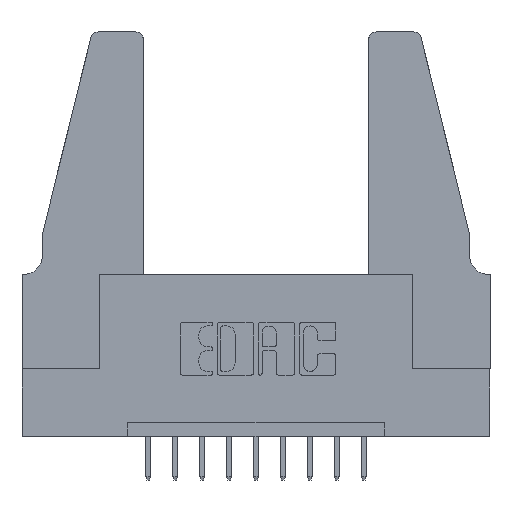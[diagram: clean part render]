
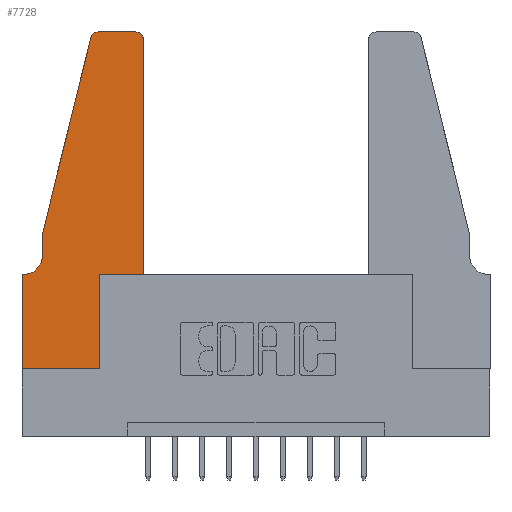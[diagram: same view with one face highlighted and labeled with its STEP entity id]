
A CAD part, top view. The second image highlights one B-rep face of the part: STEP entity #7728.
In plain terms, the highlighted planar face has unit normal (0, 0, 1).
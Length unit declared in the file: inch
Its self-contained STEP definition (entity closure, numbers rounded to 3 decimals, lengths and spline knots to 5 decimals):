
#264 = LINE ( 'NONE', #12592, #4677 ) ;
#553 = AXIS2_PLACEMENT_3D ( 'NONE', #3052, #13260, #12373 ) ;
#687 = CARTESIAN_POINT ( 'NONE',  ( 0.0755, 0.35, 0.37 ) ) ;
#752 = DIRECTION ( 'NONE',  ( 1., 0., 0. ) ) ;
#767 = EDGE_CURVE ( 'NONE', #12014, #10453, #8847, .T. ) ;
#800 = DIRECTION ( 'NONE',  ( -1., 0., 0. ) ) ;
#959 = CIRCLE ( 'NONE', #2116, 0.03 ) ;
#1011 = CIRCLE ( 'NONE', #4872, 0.07 ) ;
#1064 = EDGE_CURVE ( 'NONE', #10390, #3159, #1011, .T. ) ;
#1128 = DIRECTION ( 'NONE',  ( 0., -1., 0. ) ) ;
#1239 = LINE ( 'NONE', #7819, #7408 ) ;
#1269 = EDGE_CURVE ( 'NONE', #4932, #11868, #3289, .T. ) ;
#1440 = VERTEX_POINT ( 'NONE', #8044 ) ;
#1681 = CARTESIAN_POINT ( 'NONE',  ( 0.0755, 0.5, 0.37 ) ) ;
#1731 = CARTESIAN_POINT ( 'NONE',  ( 0.284, 1.25, 0.37 ) ) ;
#1880 = ORIENTED_EDGE ( 'NONE', *, *, #13089, .T. ) ;
#1956 = EDGE_LOOP ( 'NONE', ( #6369, #12515, #7889, #10218, #8423, #2239, #7004, #12622, #2029, #1880, #2650, #7064 ) ) ;
#2029 = ORIENTED_EDGE ( 'NONE', *, *, #767, .T. ) ;
#2116 = AXIS2_PLACEMENT_3D ( 'NONE', #11797, #7597, #5550 ) ;
#2181 = DIRECTION ( 'NONE',  ( -1., 0., 0. ) ) ;
#2197 = EDGE_CURVE ( 'NONE', #4420, #4932, #9110, .T. ) ;
#2239 = ORIENTED_EDGE ( 'NONE', *, *, #7459, .T. ) ;
#2402 = LINE ( 'NONE', #2996, #12464 ) ;
#2503 = VERTEX_POINT ( 'NONE', #6435 ) ;
#2626 = FACE_OUTER_BOUND ( 'NONE', #1956, .T. ) ;
#2650 = ORIENTED_EDGE ( 'NONE', *, *, #4150, .T. ) ;
#2946 = EDGE_CURVE ( 'NONE', #3997, #10234, #959, .T. ) ;
#2996 = CARTESIAN_POINT ( 'NONE',  ( 0.2605, 1.25, 0.37 ) ) ;
#3052 = CARTESIAN_POINT ( 'NONE',  ( 0.284, 1.22, 0.37 ) ) ;
#3159 = VERTEX_POINT ( 'NONE', #6790 ) ;
#3221 = CARTESIAN_POINT ( 'NONE',  ( 0.0055, 0.42, 0.37 ) ) ;
#3289 = LINE ( 'NONE', #1681, #3919 ) ;
#3467 = DIRECTION ( 'NONE',  ( 0., 1., 0. ) ) ;
#3749 = DIRECTION ( 'NONE',  ( 1., 0., 0. ) ) ;
#3885 = LINE ( 'NONE', #3972, #10053 ) ;
#3919 = VECTOR ( 'NONE', #4804, 39.37008 ) ;
#3972 = CARTESIAN_POINT ( 'NONE',  ( 0., 0., 0.37 ) ) ;
#3997 = VERTEX_POINT ( 'NONE', #8979 ) ;
#4150 = EDGE_CURVE ( 'NONE', #1440, #3997, #264, .T. ) ;
#4194 = PLANE ( 'NONE',  #8850 ) ;
#4245 = DIRECTION ( 'NONE',  ( 0., 0., -1. ) ) ;
#4420 = VERTEX_POINT ( 'NONE', #1731 ) ;
#4478 = EDGE_CURVE ( 'NONE', #11868, #10390, #1239, .T. ) ;
#4579 = EDGE_CURVE ( 'NONE', #10234, #4420, #2402, .T. ) ;
#4677 = VECTOR ( 'NONE', #8493, 39.37008 ) ;
#4792 = VECTOR ( 'NONE', #1128, 39.37008 ) ;
#4804 = DIRECTION ( 'NONE',  ( -0.239, -0.971, 0. ) ) ;
#4859 = CARTESIAN_POINT ( 'NONE',  ( 0.2865, 0., 0.37 ) ) ;
#4872 = AXIS2_PLACEMENT_3D ( 'NONE', #3221, #4245, #2181 ) ;
#4932 = VERTEX_POINT ( 'NONE', #9195 ) ;
#5506 = CARTESIAN_POINT ( 'NONE',  ( 0.0755, 0.42, 0.37 ) ) ;
#5550 = DIRECTION ( 'NONE',  ( 1., 0., 0. ) ) ;
#6369 = ORIENTED_EDGE ( 'NONE', *, *, #4579, .T. ) ;
#6435 = CARTESIAN_POINT ( 'NONE',  ( 0., 0., 0.37 ) ) ;
#6579 = EDGE_CURVE ( 'NONE', #7471, #2503, #8677, .T. ) ;
#6692 = CARTESIAN_POINT ( 'NONE',  ( 0.2865, 0.35, 0.37 ) ) ;
#6694 = LINE ( 'NONE', #11134, #9611 ) ;
#6790 = CARTESIAN_POINT ( 'NONE',  ( 0.0055, 0.35, 0.37 ) ) ;
#7004 = ORIENTED_EDGE ( 'NONE', *, *, #6579, .T. ) ;
#7064 = ORIENTED_EDGE ( 'NONE', *, *, #2946, .T. ) ;
#7071 = CARTESIAN_POINT ( 'NONE',  ( 0.4205, 1.25, 0.37 ) ) ;
#7408 = VECTOR ( 'NONE', #9173, 39.37008 ) ;
#7459 = EDGE_CURVE ( 'NONE', #3159, #7471, #12400, .T. ) ;
#7471 = VERTEX_POINT ( 'NONE', #11082 ) ;
#7597 = DIRECTION ( 'NONE',  ( 0., 0., 1. ) ) ;
#7685 = EDGE_CURVE ( 'NONE', #2503, #12014, #3885, .T. ) ;
#7728 = ADVANCED_FACE ( 'NONE', ( #2626 ), #4194, .T. ) ;
#7819 = CARTESIAN_POINT ( 'NONE',  ( 0.0755, 0.5, 0.37 ) ) ;
#7889 = ORIENTED_EDGE ( 'NONE', *, *, #1269, .T. ) ;
#8044 = CARTESIAN_POINT ( 'NONE',  ( 0.4505, 0.35, 0.37 ) ) ;
#8134 = VECTOR ( 'NONE', #11125, 39.37008 ) ;
#8423 = ORIENTED_EDGE ( 'NONE', *, *, #1064, .T. ) ;
#8493 = DIRECTION ( 'NONE',  ( 0., 1., 0. ) ) ;
#8677 = LINE ( 'NONE', #10558, #4792 ) ;
#8847 = LINE ( 'NONE', #6692, #10595 ) ;
#8850 = AXIS2_PLACEMENT_3D ( 'NONE', #10308, #13415, #11478 ) ;
#8979 = CARTESIAN_POINT ( 'NONE',  ( 0.4505, 1.22, 0.37 ) ) ;
#9110 = CIRCLE ( 'NONE', #553, 0.03 ) ;
#9173 = DIRECTION ( 'NONE',  ( 0., -1., 0. ) ) ;
#9195 = CARTESIAN_POINT ( 'NONE',  ( 0.25487, 1.22718, 0.37 ) ) ;
#9611 = VECTOR ( 'NONE', #3749, 39.37008 ) ;
#10053 = VECTOR ( 'NONE', #752, 39.37008 ) ;
#10218 = ORIENTED_EDGE ( 'NONE', *, *, #4478, .T. ) ;
#10234 = VERTEX_POINT ( 'NONE', #7071 ) ;
#10308 = CARTESIAN_POINT ( 'NONE',  ( 0., 0.35, 0.37 ) ) ;
#10390 = VERTEX_POINT ( 'NONE', #5506 ) ;
#10453 = VERTEX_POINT ( 'NONE', #10675 ) ;
#10558 = CARTESIAN_POINT ( 'NONE',  ( 0., 0., 0.37 ) ) ;
#10595 = VECTOR ( 'NONE', #3467, 39.37008 ) ;
#10675 = CARTESIAN_POINT ( 'NONE',  ( 0.2865, 0.35, 0.37 ) ) ;
#11082 = CARTESIAN_POINT ( 'NONE',  ( 0., 0.35, 0.37 ) ) ;
#11125 = DIRECTION ( 'NONE',  ( -1., 0., 0. ) ) ;
#11134 = CARTESIAN_POINT ( 'NONE',  ( 0.4505, 0.35, 0.37 ) ) ;
#11478 = DIRECTION ( 'NONE',  ( 1., 0., 0. ) ) ;
#11797 = CARTESIAN_POINT ( 'NONE',  ( 0.4205, 1.22, 0.37 ) ) ;
#11868 = VERTEX_POINT ( 'NONE', #12097 ) ;
#12014 = VERTEX_POINT ( 'NONE', #4859 ) ;
#12097 = CARTESIAN_POINT ( 'NONE',  ( 0.0755, 0.5, 0.37 ) ) ;
#12373 = DIRECTION ( 'NONE',  ( 1., 0., 0. ) ) ;
#12400 = LINE ( 'NONE', #687, #8134 ) ;
#12464 = VECTOR ( 'NONE', #800, 39.37008 ) ;
#12515 = ORIENTED_EDGE ( 'NONE', *, *, #2197, .T. ) ;
#12592 = CARTESIAN_POINT ( 'NONE',  ( 0.4505, 0.35, 0.37 ) ) ;
#12622 = ORIENTED_EDGE ( 'NONE', *, *, #7685, .T. ) ;
#13089 = EDGE_CURVE ( 'NONE', #10453, #1440, #6694, .T. ) ;
#13260 = DIRECTION ( 'NONE',  ( 0., 0., 1. ) ) ;
#13415 = DIRECTION ( 'NONE',  ( 0., 0., 1. ) ) ;
